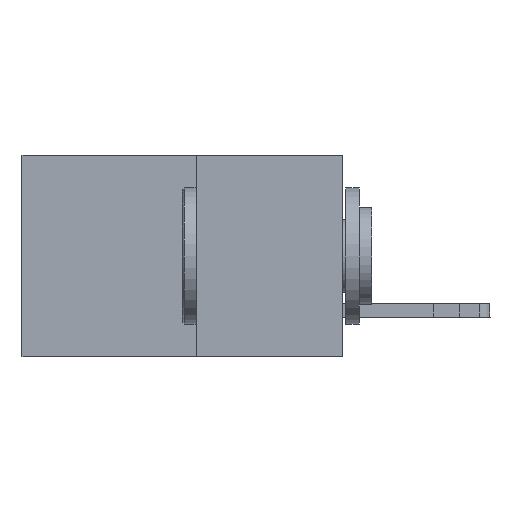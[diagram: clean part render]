
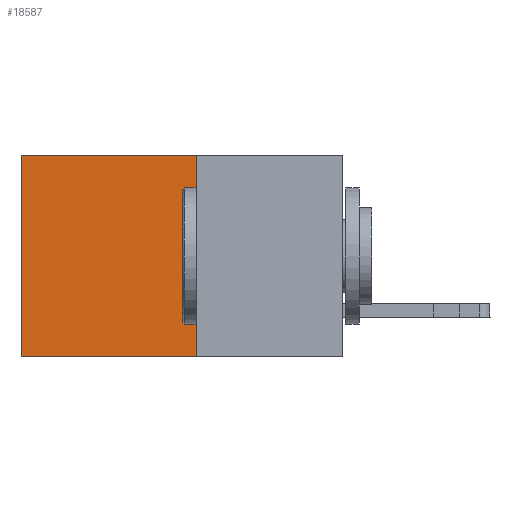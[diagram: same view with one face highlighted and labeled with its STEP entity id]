
A CAD part, left-side view. The second image highlights one B-rep face of the part: STEP entity #18587.
In plain terms, the highlighted planar face has unit normal (-1, 0, 0).
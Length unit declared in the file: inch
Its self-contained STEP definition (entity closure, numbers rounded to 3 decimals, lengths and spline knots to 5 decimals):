
#607 = AXIS2_PLACEMENT_3D ( 'NONE', #20698, #15293, #8745 ) ;
#656 = CARTESIAN_POINT ( 'NONE',  ( 0.277, 0.27, -0.37 ) ) ;
#854 = VERTEX_POINT ( 'NONE', #14645 ) ;
#924 = DIRECTION ( 'NONE',  ( 0., 0., -1. ) ) ;
#2317 = LINE ( 'NONE', #656, #18122 ) ;
#2321 = EDGE_CURVE ( 'NONE', #3563, #10518, #20495, .T. ) ;
#2572 = VECTOR ( 'NONE', #924, 39.37008 ) ;
#3563 = VERTEX_POINT ( 'NONE', #13168 ) ;
#3906 = PLANE ( 'NONE',  #607 ) ;
#4021 = VECTOR ( 'NONE', #13750, 39.37008 ) ;
#4123 = LINE ( 'NONE', #9208, #20942 ) ;
#4458 = DIRECTION ( 'NONE',  ( 0., 1., 0. ) ) ;
#5175 = EDGE_CURVE ( 'NONE', #10412, #854, #4123, .T. ) ;
#7355 = DIRECTION ( 'NONE',  ( 0., 0., -1. ) ) ;
#8691 = CARTESIAN_POINT ( 'NONE',  ( 0.277, 0.27, 0. ) ) ;
#8745 = DIRECTION ( 'NONE',  ( 0., 0., -1. ) ) ;
#8992 = EDGE_LOOP ( 'NONE', ( #18081, #20023, #15088, #11711 ) ) ;
#9208 = CARTESIAN_POINT ( 'NONE',  ( 0.277, 0.27, 0. ) ) ;
#9488 = CARTESIAN_POINT ( 'NONE',  ( 0.277, 0.59, -0.37 ) ) ;
#10412 = VERTEX_POINT ( 'NONE', #8691 ) ;
#10518 = VERTEX_POINT ( 'NONE', #10575 ) ;
#10575 = CARTESIAN_POINT ( 'NONE',  ( 0.277, 0.59, -0.37 ) ) ;
#11711 = ORIENTED_EDGE ( 'NONE', *, *, #5175, .T. ) ;
#13168 = CARTESIAN_POINT ( 'NONE',  ( 0.277, 0.27, -0.37 ) ) ;
#13626 = FACE_OUTER_BOUND ( 'NONE', #8992, .T. ) ;
#13750 = DIRECTION ( 'NONE',  ( 0., 1., 0. ) ) ;
#14606 = EDGE_CURVE ( 'NONE', #10412, #3563, #2317, .T. ) ;
#14645 = CARTESIAN_POINT ( 'NONE',  ( 0.277, 0.59, 0. ) ) ;
#15088 = ORIENTED_EDGE ( 'NONE', *, *, #14606, .F. ) ;
#15293 = DIRECTION ( 'NONE',  ( 1., 0., 0. ) ) ;
#15729 = CARTESIAN_POINT ( 'NONE',  ( 0.277, 0.27, -0.37 ) ) ;
#18081 = ORIENTED_EDGE ( 'NONE', *, *, #20018, .T. ) ;
#18122 = VECTOR ( 'NONE', #7355, 39.37008 ) ;
#18587 = ADVANCED_FACE ( 'NONE', ( #13626 ), #3906, .F. ) ;
#19460 = LINE ( 'NONE', #9488, #2572 ) ;
#20018 = EDGE_CURVE ( 'NONE', #854, #10518, #19460, .T. ) ;
#20023 = ORIENTED_EDGE ( 'NONE', *, *, #2321, .F. ) ;
#20495 = LINE ( 'NONE', #15729, #4021 ) ;
#20698 = CARTESIAN_POINT ( 'NONE',  ( 0.277, 0.27, -0.37 ) ) ;
#20942 = VECTOR ( 'NONE', #4458, 39.37008 ) ;
